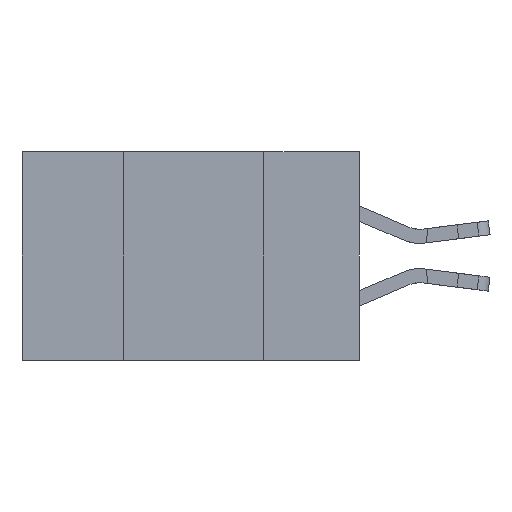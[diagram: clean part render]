
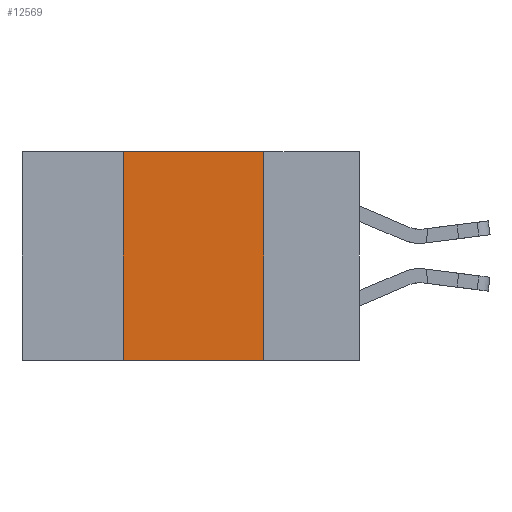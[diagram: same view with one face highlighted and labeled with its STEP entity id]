
A CAD part, left-side view. The second image highlights one B-rep face of the part: STEP entity #12569.
In plain terms, the highlighted planar face has unit normal (-1, 0, 0).
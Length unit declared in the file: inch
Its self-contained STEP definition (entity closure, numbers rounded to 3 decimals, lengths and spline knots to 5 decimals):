
#407 = CARTESIAN_POINT ( 'NONE',  ( 0., 0.6, 0. ) ) ;
#551 = ORIENTED_EDGE ( 'NONE', *, *, #8855, .F. ) ;
#1896 = CARTESIAN_POINT ( 'NONE',  ( 0., 0.6, 0. ) ) ;
#2067 = CARTESIAN_POINT ( 'NONE',  ( 0., 0.17, 0. ) ) ;
#2081 = DIRECTION ( 'NONE',  ( 0., 0., 1. ) ) ;
#2874 = LINE ( 'NONE', #407, #13875 ) ;
#3750 = ORIENTED_EDGE ( 'NONE', *, *, #27636, .F. ) ;
#3929 = VERTEX_POINT ( 'NONE', #24989 ) ;
#4174 = DIRECTION ( 'NONE',  ( 1., 0., 0. ) ) ;
#4260 = VERTEX_POINT ( 'NONE', #23753 ) ;
#4533 = LINE ( 'NONE', #26811, #16160 ) ;
#4921 = VERTEX_POINT ( 'NONE', #2067 ) ;
#7087 = FACE_OUTER_BOUND ( 'NONE', #25207, .T. ) ;
#8855 = EDGE_CURVE ( 'NONE', #21783, #3929, #12165, .T. ) ;
#8975 = EDGE_CURVE ( 'NONE', #3929, #4921, #2874, .T. ) ;
#9485 = DIRECTION ( 'NONE',  ( 0., -1., 0. ) ) ;
#12165 = LINE ( 'NONE', #28100, #22899 ) ;
#12569 = ADVANCED_FACE ( 'NONE', ( #7087 ), #27823, .F. ) ;
#13286 = AXIS2_PLACEMENT_3D ( 'NONE', #1896, #4174, #19421 ) ;
#13875 = VECTOR ( 'NONE', #18001, 39.37008 ) ;
#14046 = DIRECTION ( 'NONE',  ( 0., 0., -1. ) ) ;
#14910 = VECTOR ( 'NONE', #9485, 39.37008 ) ;
#15377 = ORIENTED_EDGE ( 'NONE', *, *, #8975, .F. ) ;
#16160 = VECTOR ( 'NONE', #14046, 39.37008 ) ;
#18001 = DIRECTION ( 'NONE',  ( 0., -1., 0. ) ) ;
#19421 = DIRECTION ( 'NONE',  ( 0., 0., -1. ) ) ;
#19433 = ORIENTED_EDGE ( 'NONE', *, *, #25594, .T. ) ;
#20621 = LINE ( 'NONE', #24605, #14910 ) ;
#21783 = VERTEX_POINT ( 'NONE', #24276 ) ;
#22899 = VECTOR ( 'NONE', #2081, 39.37008 ) ;
#23753 = CARTESIAN_POINT ( 'NONE',  ( 0., 0.17, -0.37 ) ) ;
#24276 = CARTESIAN_POINT ( 'NONE',  ( 0., 0.42, -0.37 ) ) ;
#24605 = CARTESIAN_POINT ( 'NONE',  ( 0., 0.6, -0.37 ) ) ;
#24989 = CARTESIAN_POINT ( 'NONE',  ( 0., 0.42, 0. ) ) ;
#25207 = EDGE_LOOP ( 'NONE', ( #3750, #15377, #551, #19433 ) ) ;
#25594 = EDGE_CURVE ( 'NONE', #21783, #4260, #20621, .T. ) ;
#26811 = CARTESIAN_POINT ( 'NONE',  ( 0., 0.17, 0. ) ) ;
#27636 = EDGE_CURVE ( 'NONE', #4921, #4260, #4533, .T. ) ;
#27823 = PLANE ( 'NONE',  #13286 ) ;
#28100 = CARTESIAN_POINT ( 'NONE',  ( 0., 0.42, 0. ) ) ;
